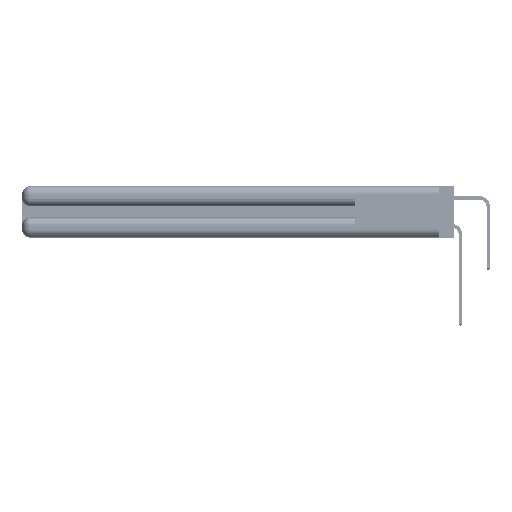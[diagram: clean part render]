
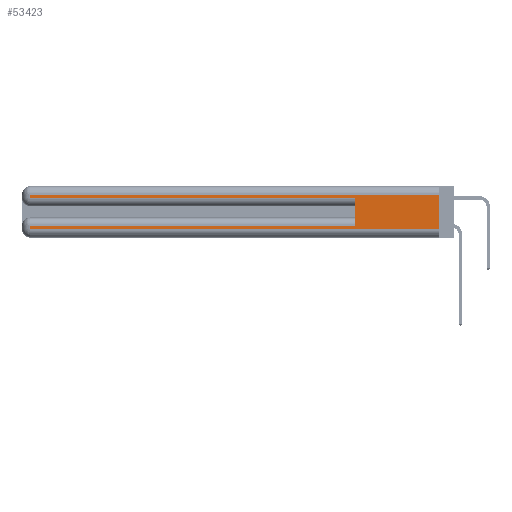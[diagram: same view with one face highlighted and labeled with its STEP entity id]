
A CAD part, left-side view. The second image highlights one B-rep face of the part: STEP entity #53423.
In plain terms, the highlighted planar face has unit normal (-1, 0, 0).
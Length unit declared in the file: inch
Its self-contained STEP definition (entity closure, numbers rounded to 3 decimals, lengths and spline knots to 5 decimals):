
#413 = LINE ( 'NONE', #12624, #10203 ) ;
#1198 = CARTESIAN_POINT ( 'NONE',  ( 0., 0., 0.37 ) ) ;
#1492 = EDGE_CURVE ( 'NONE', #17427, #31527, #21220, .T. ) ;
#2494 = VECTOR ( 'NONE', #13474, 39.37008 ) ;
#4067 = CARTESIAN_POINT ( 'NONE',  ( 0., 0.6, 0.145 ) ) ;
#5319 = EDGE_CURVE ( 'NONE', #49070, #21170, #27386, .T. ) ;
#6019 = VECTOR ( 'NONE', #13763, 39.37008 ) ;
#7543 = DIRECTION ( 'NONE',  ( 1., 0., 0. ) ) ;
#7631 = DIRECTION ( 'NONE',  ( 0., 1., 0. ) ) ;
#8237 = ORIENTED_EDGE ( 'NONE', *, *, #26841, .T. ) ;
#8388 = VERTEX_POINT ( 'NONE', #35631 ) ;
#8454 = DIRECTION ( 'NONE',  ( 0., 1., 0. ) ) ;
#9483 = VERTEX_POINT ( 'NONE', #26680 ) ;
#10203 = VECTOR ( 'NONE', #8454, 39.37008 ) ;
#11018 = FACE_OUTER_BOUND ( 'NONE', #28215, .T. ) ;
#12165 = CARTESIAN_POINT ( 'NONE',  ( 0., 2.94, 0.37 ) ) ;
#12427 = DIRECTION ( 'NONE',  ( 0., 0., 1. ) ) ;
#12624 = CARTESIAN_POINT ( 'NONE',  ( 0., 0., 0.085 ) ) ;
#12895 = VECTOR ( 'NONE', #30918, 39.37008 ) ;
#13474 = DIRECTION ( 'NONE',  ( 0., 0., -1. ) ) ;
#13539 = LINE ( 'NONE', #17436, #2494 ) ;
#13763 = DIRECTION ( 'NONE',  ( 0., 0., -1. ) ) ;
#14004 = EDGE_CURVE ( 'NONE', #9483, #31579, #51286, .T. ) ;
#14062 = ORIENTED_EDGE ( 'NONE', *, *, #14004, .F. ) ;
#15314 = DIRECTION ( 'NONE',  ( 0., -1., 0. ) ) ;
#16382 = VECTOR ( 'NONE', #12427, 39.37008 ) ;
#17162 = EDGE_CURVE ( 'NONE', #31527, #31579, #42546, .T. ) ;
#17427 = VERTEX_POINT ( 'NONE', #29194 ) ;
#17436 = CARTESIAN_POINT ( 'NONE',  ( 0., 2.94, 0.37 ) ) ;
#18594 = CARTESIAN_POINT ( 'NONE',  ( 0., 0., 0.285 ) ) ;
#18600 = ORIENTED_EDGE ( 'NONE', *, *, #17162, .T. ) ;
#19728 = CARTESIAN_POINT ( 'NONE',  ( 0., 2.94, 0.31 ) ) ;
#19949 = CARTESIAN_POINT ( 'NONE',  ( 0., 0., 0.31 ) ) ;
#21170 = VERTEX_POINT ( 'NONE', #35698 ) ;
#21220 = LINE ( 'NONE', #12165, #41918 ) ;
#23448 = VECTOR ( 'NONE', #7631, 39.37008 ) ;
#24102 = VERTEX_POINT ( 'NONE', #19728 ) ;
#24416 = ORIENTED_EDGE ( 'NONE', *, *, #27560, .T. ) ;
#26680 = CARTESIAN_POINT ( 'NONE',  ( 0., 0., 0.31 ) ) ;
#26841 = EDGE_CURVE ( 'NONE', #24102, #8388, #13539, .T. ) ;
#27386 = LINE ( 'NONE', #4067, #16382 ) ;
#27560 = EDGE_CURVE ( 'NONE', #49070, #17427, #413, .T. ) ;
#28215 = EDGE_LOOP ( 'NONE', ( #14062, #43835, #8237, #50903, #39952, #24416, #39310, #18600 ) ) ;
#29194 = CARTESIAN_POINT ( 'NONE',  ( 0., 2.94, 0.085 ) ) ;
#30918 = DIRECTION ( 'NONE',  ( 0., -1., 0. ) ) ;
#31527 = VERTEX_POINT ( 'NONE', #52918 ) ;
#31579 = VERTEX_POINT ( 'NONE', #48958 ) ;
#32322 = PLANE ( 'NONE',  #47002 ) ;
#32765 = DIRECTION ( 'NONE',  ( 0., 0., -1. ) ) ;
#35631 = CARTESIAN_POINT ( 'NONE',  ( 0., 2.94, 0.285 ) ) ;
#35698 = CARTESIAN_POINT ( 'NONE',  ( 0., 0.6, 0.285 ) ) ;
#36170 = EDGE_CURVE ( 'NONE', #9483, #24102, #45435, .T. ) ;
#36473 = DIRECTION ( 'NONE',  ( 0., 0., -1. ) ) ;
#39310 = ORIENTED_EDGE ( 'NONE', *, *, #1492, .T. ) ;
#39952 = ORIENTED_EDGE ( 'NONE', *, *, #5319, .F. ) ;
#40076 = CARTESIAN_POINT ( 'NONE',  ( 0., 0., 0.06 ) ) ;
#40684 = EDGE_CURVE ( 'NONE', #8388, #21170, #48472, .T. ) ;
#41918 = VECTOR ( 'NONE', #32765, 39.37008 ) ;
#42546 = LINE ( 'NONE', #40076, #53508 ) ;
#43835 = ORIENTED_EDGE ( 'NONE', *, *, #36170, .T. ) ;
#44613 = CARTESIAN_POINT ( 'NONE',  ( 0., 0., 0.37 ) ) ;
#45435 = LINE ( 'NONE', #19949, #23448 ) ;
#47002 = AXIS2_PLACEMENT_3D ( 'NONE', #44613, #7543, #36473 ) ;
#48472 = LINE ( 'NONE', #18594, #12895 ) ;
#48958 = CARTESIAN_POINT ( 'NONE',  ( 0., 0., 0.06 ) ) ;
#49070 = VERTEX_POINT ( 'NONE', #52230 ) ;
#50903 = ORIENTED_EDGE ( 'NONE', *, *, #40684, .T. ) ;
#51286 = LINE ( 'NONE', #1198, #6019 ) ;
#52230 = CARTESIAN_POINT ( 'NONE',  ( 0., 0.6, 0.085 ) ) ;
#52918 = CARTESIAN_POINT ( 'NONE',  ( 0., 2.94, 0.06 ) ) ;
#53423 = ADVANCED_FACE ( 'NONE', ( #11018 ), #32322, .F. ) ;
#53508 = VECTOR ( 'NONE', #15314, 39.37008 ) ;
